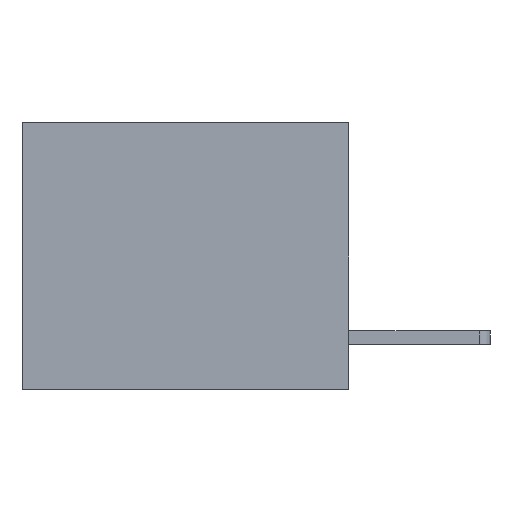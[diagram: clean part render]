
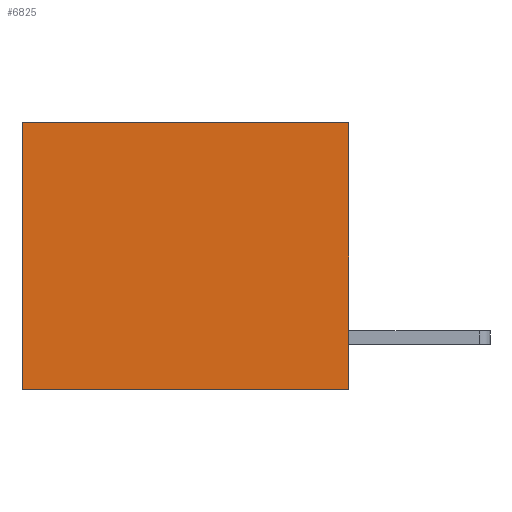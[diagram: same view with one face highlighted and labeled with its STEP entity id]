
A CAD part, left-side view. The second image highlights one B-rep face of the part: STEP entity #6825.
In plain terms, the highlighted planar face has unit normal (-1, 0, 0).
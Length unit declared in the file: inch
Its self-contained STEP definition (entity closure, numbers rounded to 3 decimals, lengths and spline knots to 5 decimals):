
#9 = DIRECTION ( 'NONE',  ( 0., 0., -1. ) ) ;
#610 = EDGE_CURVE ( 'NONE', #4793, #4333, #5894, .T. ) ;
#977 = DIRECTION ( 'NONE',  ( 0., 1., 0. ) ) ;
#1893 = EDGE_LOOP ( 'NONE', ( #7751, #5707, #4372, #3708 ) ) ;
#2379 = EDGE_CURVE ( 'NONE', #3101, #4333, #3021, .T. ) ;
#2442 = VECTOR ( 'NONE', #6314, 39.37008 ) ;
#2462 = CARTESIAN_POINT ( 'NONE',  ( 0.3165, 0.6, -0.49 ) ) ;
#2538 = AXIS2_PLACEMENT_3D ( 'NONE', #7982, #4357, #9 ) ;
#2819 = CARTESIAN_POINT ( 'NONE',  ( 0.3165, 0., -0.49 ) ) ;
#2995 = EDGE_CURVE ( 'NONE', #3399, #4793, #6636, .T. ) ;
#3021 = LINE ( 'NONE', #8103, #3704 ) ;
#3076 = DIRECTION ( 'NONE',  ( 0., 0., -1. ) ) ;
#3101 = VERTEX_POINT ( 'NONE', #9217 ) ;
#3399 = VERTEX_POINT ( 'NONE', #5170 ) ;
#3516 = CARTESIAN_POINT ( 'NONE',  ( 0.3165, 0., -0.49 ) ) ;
#3620 = PLANE ( 'NONE',  #2538 ) ;
#3704 = VECTOR ( 'NONE', #3076, 39.37008 ) ;
#3708 = ORIENTED_EDGE ( 'NONE', *, *, #4002, .T. ) ;
#4002 = EDGE_CURVE ( 'NONE', #3399, #3101, #7545, .T. ) ;
#4333 = VERTEX_POINT ( 'NONE', #2462 ) ;
#4357 = DIRECTION ( 'NONE',  ( 1., 0., 0. ) ) ;
#4372 = ORIENTED_EDGE ( 'NONE', *, *, #2995, .F. ) ;
#4707 = FACE_OUTER_BOUND ( 'NONE', #1893, .T. ) ;
#4793 = VERTEX_POINT ( 'NONE', #3516 ) ;
#5110 = VECTOR ( 'NONE', #977, 39.37008 ) ;
#5170 = CARTESIAN_POINT ( 'NONE',  ( 0.3165, 0., 0. ) ) ;
#5707 = ORIENTED_EDGE ( 'NONE', *, *, #610, .F. ) ;
#5894 = LINE ( 'NONE', #6696, #5110 ) ;
#6314 = DIRECTION ( 'NONE',  ( 0., 0., -1. ) ) ;
#6636 = LINE ( 'NONE', #2819, #2442 ) ;
#6696 = CARTESIAN_POINT ( 'NONE',  ( 0.3165, 0., -0.49 ) ) ;
#6825 = ADVANCED_FACE ( 'NONE', ( #4707 ), #3620, .F. ) ;
#7414 = VECTOR ( 'NONE', #7908, 39.37008 ) ;
#7545 = LINE ( 'NONE', #8608, #7414 ) ;
#7751 = ORIENTED_EDGE ( 'NONE', *, *, #2379, .T. ) ;
#7908 = DIRECTION ( 'NONE',  ( 0., 1., 0. ) ) ;
#7982 = CARTESIAN_POINT ( 'NONE',  ( 0.3165, 0., -0.49 ) ) ;
#8103 = CARTESIAN_POINT ( 'NONE',  ( 0.3165, 0.6, -0.49 ) ) ;
#8608 = CARTESIAN_POINT ( 'NONE',  ( 0.3165, 0., 0. ) ) ;
#9217 = CARTESIAN_POINT ( 'NONE',  ( 0.3165, 0.6, 0. ) ) ;
